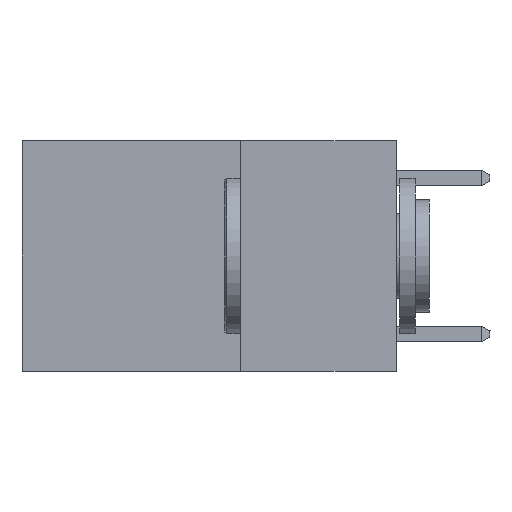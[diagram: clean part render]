
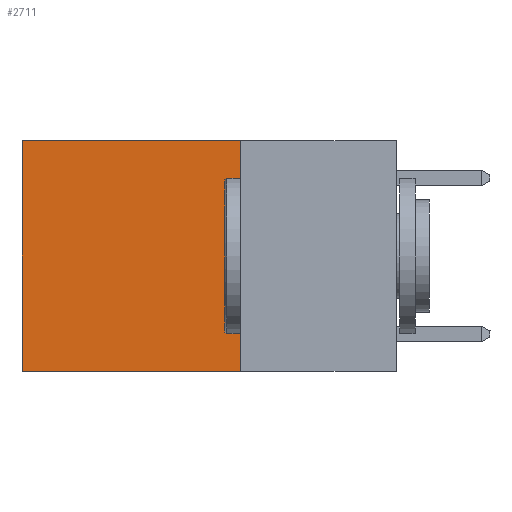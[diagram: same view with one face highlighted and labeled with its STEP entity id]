
A CAD part, left-side view. The second image highlights one B-rep face of the part: STEP entity #2711.
In plain terms, the highlighted planar face has unit normal (-1, 0, 0).
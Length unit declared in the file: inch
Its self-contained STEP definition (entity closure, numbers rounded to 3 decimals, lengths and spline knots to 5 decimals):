
#586 = LINE ( 'NONE', #15981, #16438 ) ;
#645 = CARTESIAN_POINT ( 'NONE',  ( 0.2625, 0.6, -0.37 ) ) ;
#833 = VERTEX_POINT ( 'NONE', #645 ) ;
#2040 = ORIENTED_EDGE ( 'NONE', *, *, #13444, .T. ) ;
#2451 = CARTESIAN_POINT ( 'NONE',  ( 0.2625, 0.25, 0. ) ) ;
#2582 = CARTESIAN_POINT ( 'NONE',  ( 0.2625, 0.6, 0. ) ) ;
#2711 = ADVANCED_FACE ( 'NONE', ( #7894 ), #13519, .F. ) ;
#3655 = VERTEX_POINT ( 'NONE', #11912 ) ;
#4378 = ORIENTED_EDGE ( 'NONE', *, *, #7867, .F. ) ;
#4726 = CARTESIAN_POINT ( 'NONE',  ( 0.2625, 0.25, -0.37 ) ) ;
#5029 = VERTEX_POINT ( 'NONE', #4726 ) ;
#5915 = CARTESIAN_POINT ( 'NONE',  ( 0.2625, 0.6, 0. ) ) ;
#6202 = LINE ( 'NONE', #9305, #13169 ) ;
#7362 = VERTEX_POINT ( 'NONE', #2582 ) ;
#7867 = EDGE_CURVE ( 'NONE', #3655, #5029, #12185, .T. ) ;
#7894 = FACE_OUTER_BOUND ( 'NONE', #14503, .T. ) ;
#8854 = VECTOR ( 'NONE', #9139, 39.37008 ) ;
#9139 = DIRECTION ( 'NONE',  ( 0., 0., -1. ) ) ;
#9305 = CARTESIAN_POINT ( 'NONE',  ( 0.2625, 0.25, -0.37 ) ) ;
#9375 = CARTESIAN_POINT ( 'NONE',  ( 0.2625, 0.25, 0. ) ) ;
#9476 = DIRECTION ( 'NONE',  ( 1., 0., 0. ) ) ;
#9699 = ORIENTED_EDGE ( 'NONE', *, *, #15143, .F. ) ;
#9863 = DIRECTION ( 'NONE',  ( 0., 0., -1. ) ) ;
#10052 = LINE ( 'NONE', #5915, #16657 ) ;
#11912 = CARTESIAN_POINT ( 'NONE',  ( 0.2625, 0.25, 0. ) ) ;
#12185 = LINE ( 'NONE', #2451, #8854 ) ;
#12446 = AXIS2_PLACEMENT_3D ( 'NONE', #9375, #9476, #13616 ) ;
#13169 = VECTOR ( 'NONE', #17422, 39.37008 ) ;
#13444 = EDGE_CURVE ( 'NONE', #7362, #833, #10052, .T. ) ;
#13519 = PLANE ( 'NONE',  #12446 ) ;
#13616 = DIRECTION ( 'NONE',  ( 0., 0., -1. ) ) ;
#14390 = DIRECTION ( 'NONE',  ( 0., 1., 0. ) ) ;
#14503 = EDGE_LOOP ( 'NONE', ( #2040, #9699, #4378, #17256 ) ) ;
#15143 = EDGE_CURVE ( 'NONE', #5029, #833, #6202, .T. ) ;
#15981 = CARTESIAN_POINT ( 'NONE',  ( 0.2625, 0.25, 0. ) ) ;
#16438 = VECTOR ( 'NONE', #14390, 39.37008 ) ;
#16657 = VECTOR ( 'NONE', #9863, 39.37008 ) ;
#17256 = ORIENTED_EDGE ( 'NONE', *, *, #17714, .T. ) ;
#17422 = DIRECTION ( 'NONE',  ( 0., 1., 0. ) ) ;
#17714 = EDGE_CURVE ( 'NONE', #3655, #7362, #586, .T. ) ;
